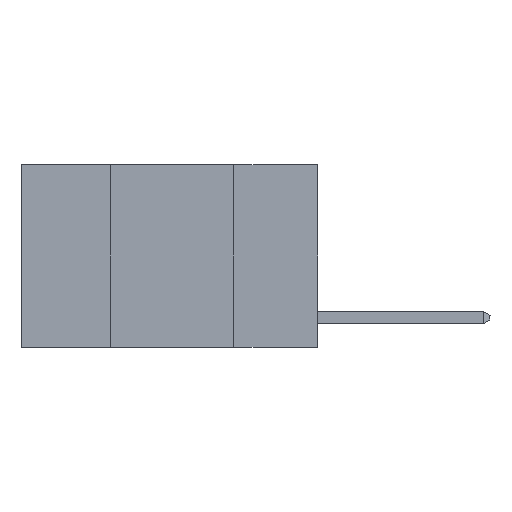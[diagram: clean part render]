
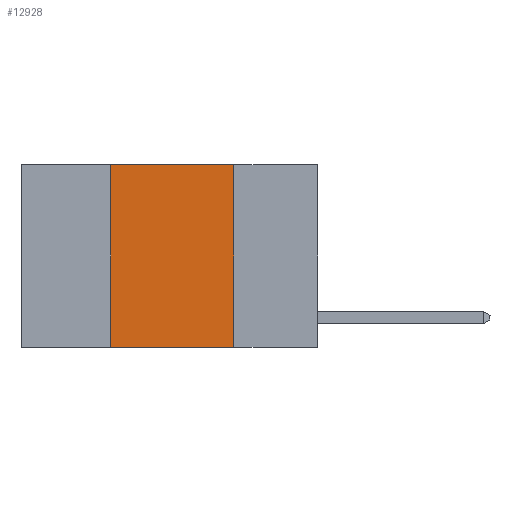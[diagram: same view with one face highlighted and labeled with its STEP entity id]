
A CAD part, left-side view. The second image highlights one B-rep face of the part: STEP entity #12928.
In plain terms, the highlighted planar face has unit normal (-1, 0, 0).
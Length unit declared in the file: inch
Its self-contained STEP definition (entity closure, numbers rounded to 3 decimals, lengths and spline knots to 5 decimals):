
#838 = LINE ( 'NONE', #13564, #9588 ) ;
#1456 = DIRECTION ( 'NONE',  ( 1., 0., 0. ) ) ;
#1968 = VERTEX_POINT ( 'NONE', #5446 ) ;
#2535 = CARTESIAN_POINT ( 'NONE',  ( 0., 0.17, 0. ) ) ;
#3812 = ORIENTED_EDGE ( 'NONE', *, *, #8422, .F. ) ;
#4223 = VERTEX_POINT ( 'NONE', #14229 ) ;
#4260 = VERTEX_POINT ( 'NONE', #13904 ) ;
#4501 = ORIENTED_EDGE ( 'NONE', *, *, #16129, .T. ) ;
#4818 = VECTOR ( 'NONE', #19647, 39.37008 ) ;
#5446 = CARTESIAN_POINT ( 'NONE',  ( 0., 0.42, 0. ) ) ;
#5994 = LINE ( 'NONE', #2535, #19268 ) ;
#8422 = EDGE_CURVE ( 'NONE', #4223, #1968, #838, .T. ) ;
#8434 = EDGE_LOOP ( 'NONE', ( #20921, #9866, #3812, #4501 ) ) ;
#8815 = EDGE_CURVE ( 'NONE', #21301, #4260, #5994, .T. ) ;
#9306 = DIRECTION ( 'NONE',  ( 0., -1., 0. ) ) ;
#9588 = VECTOR ( 'NONE', #18523, 39.37008 ) ;
#9866 = ORIENTED_EDGE ( 'NONE', *, *, #11516, .F. ) ;
#11516 = EDGE_CURVE ( 'NONE', #1968, #21301, #14386, .T. ) ;
#11583 = DIRECTION ( 'NONE',  ( 0., 0., -1. ) ) ;
#11806 = PLANE ( 'NONE',  #15382 ) ;
#12329 = LINE ( 'NONE', #20640, #13328 ) ;
#12766 = DIRECTION ( 'NONE',  ( 0., 0., -1. ) ) ;
#12928 = ADVANCED_FACE ( 'NONE', ( #18280 ), #11806, .F. ) ;
#13328 = VECTOR ( 'NONE', #9306, 39.37008 ) ;
#13564 = CARTESIAN_POINT ( 'NONE',  ( 0., 0.42, 0. ) ) ;
#13904 = CARTESIAN_POINT ( 'NONE',  ( 0., 0.17, -0.37 ) ) ;
#14229 = CARTESIAN_POINT ( 'NONE',  ( 0., 0.42, -0.37 ) ) ;
#14386 = LINE ( 'NONE', #15996, #4818 ) ;
#15047 = CARTESIAN_POINT ( 'NONE',  ( 0., 0.6, 0. ) ) ;
#15382 = AXIS2_PLACEMENT_3D ( 'NONE', #15047, #1456, #11583 ) ;
#15996 = CARTESIAN_POINT ( 'NONE',  ( 0., 0.6, 0. ) ) ;
#16129 = EDGE_CURVE ( 'NONE', #4223, #4260, #12329, .T. ) ;
#18280 = FACE_OUTER_BOUND ( 'NONE', #8434, .T. ) ;
#18523 = DIRECTION ( 'NONE',  ( 0., 0., 1. ) ) ;
#19268 = VECTOR ( 'NONE', #12766, 39.37008 ) ;
#19647 = DIRECTION ( 'NONE',  ( 0., -1., 0. ) ) ;
#20640 = CARTESIAN_POINT ( 'NONE',  ( 0., 0.6, -0.37 ) ) ;
#20921 = ORIENTED_EDGE ( 'NONE', *, *, #8815, .F. ) ;
#21028 = CARTESIAN_POINT ( 'NONE',  ( 0., 0.17, 0. ) ) ;
#21301 = VERTEX_POINT ( 'NONE', #21028 ) ;
